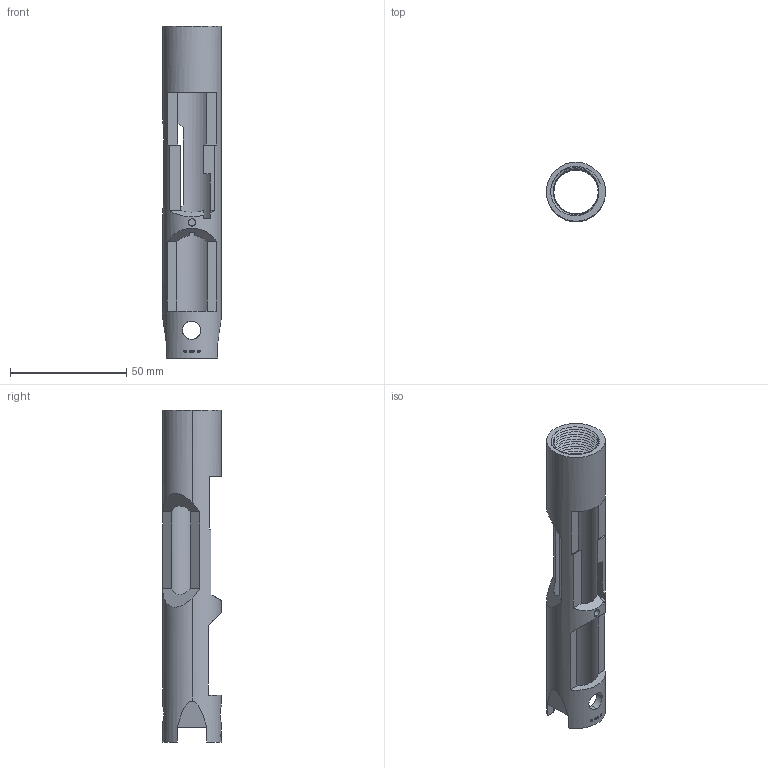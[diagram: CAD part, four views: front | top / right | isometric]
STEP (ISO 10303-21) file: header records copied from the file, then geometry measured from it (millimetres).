
FILE_DESCRIPTION (( 'STEP AP214' ), '1' );
FILE_NAME ('rugermkII.STEP', '2019-04-09T08:50:48', ( '' ), ( '' ), 'SwSTEP 2.0', 'SolidWorks 2018', '' );
FILE_SCHEMA (( 'AUTOMOTIVE_DESIGN' ));
Length unit declared in the file: inch
Products named in the file (1): rugermkII
Bounding box: 25.4 x 25.4 x 142.93 mm (x, y, z)
Volume: 22681.4 mm3; surface area: 18039.4 mm2
Topology: 1 solids, 1 shells, 112 faces, 312 edges, 206 vertices
Faces by surface type: bspline 57, plane 38, cylinder 17
Entity records: 9381 total; most frequent: CARTESIAN_POINT 7001, ORIENTED_EDGE 624, EDGE_CURVE 312, DIRECTION 252, VERTEX_POINT 206, B_SPLINE_CURVE_WITH_KNOTS 177, EDGE_LOOP 130, ADVANCED_FACE 112
